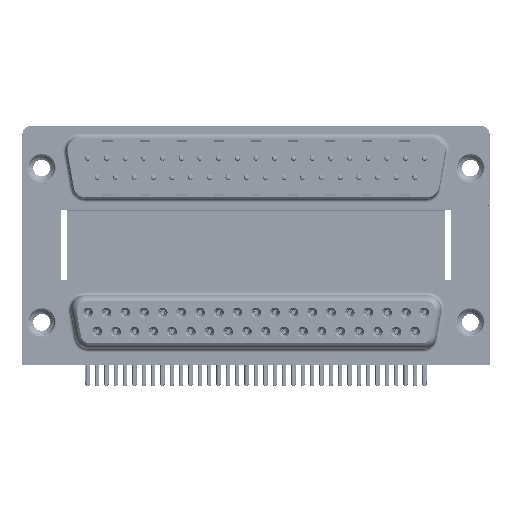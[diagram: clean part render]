
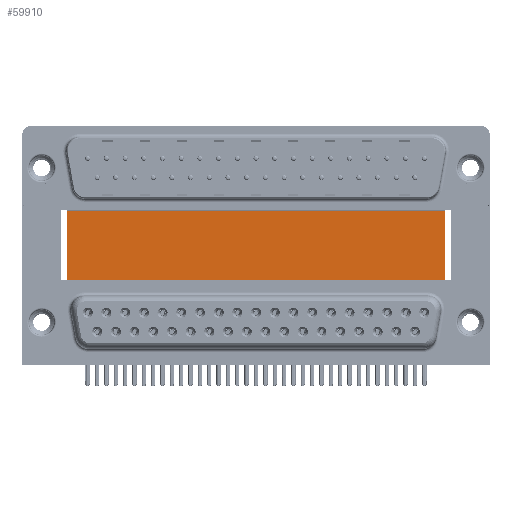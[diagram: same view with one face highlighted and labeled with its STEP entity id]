
A CAD part, top view. The second image highlights one B-rep face of the part: STEP entity #59910.
In plain terms, the highlighted planar face has unit normal (0, 0, 1).
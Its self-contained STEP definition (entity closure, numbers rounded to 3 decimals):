
#2184 = EDGE_CURVE ( 'NONE', #16338, #67508, #48367, .T. ) ;
#2792 = PLANE ( 'NONE',  #22619 ) ;
#4740 = VECTOR ( 'NONE', #37841, 1000. ) ;
#6722 = VECTOR ( 'NONE', #44417, 1000. ) ;
#8846 = DIRECTION ( 'NONE',  ( 0., 0., -1. ) ) ;
#11125 = ORIENTED_EDGE ( 'NONE', *, *, #2184, .F. ) ;
#14755 = EDGE_LOOP ( 'NONE', ( #58675, #37322, #11125, #35651 ) ) ;
#16338 = VERTEX_POINT ( 'NONE', #57147 ) ;
#21140 = LINE ( 'NONE', #42816, #4740 ) ;
#22619 = AXIS2_PLACEMENT_3D ( 'NONE', #57122, #8846, #56070 ) ;
#25188 = VERTEX_POINT ( 'NONE', #70006 ) ;
#33525 = CARTESIAN_POINT ( 'NONE',  ( 59.71, 16.585, -12. ) ) ;
#35651 = ORIENTED_EDGE ( 'NONE', *, *, #64796, .T. ) ;
#37322 = ORIENTED_EDGE ( 'NONE', *, *, #51460, .F. ) ;
#37841 = DIRECTION ( 'NONE',  ( 0., -1., 0. ) ) ;
#39160 = CARTESIAN_POINT ( 'NONE',  ( 59.71, 16.585, -12. ) ) ;
#41349 = CARTESIAN_POINT ( 'NONE',  ( 3.79, -3.735, -12. ) ) ;
#42816 = CARTESIAN_POINT ( 'NONE',  ( 3.79, 16.585, -12. ) ) ;
#43095 = CARTESIAN_POINT ( 'NONE',  ( 3.79, -3.735, -12. ) ) ;
#44417 = DIRECTION ( 'NONE',  ( 1., 0., 0. ) ) ;
#46168 = EDGE_CURVE ( 'NONE', #57973, #25188, #68975, .T. ) ;
#46302 = DIRECTION ( 'NONE',  ( 1., 0., 0. ) ) ;
#48367 = LINE ( 'NONE', #64647, #6722 ) ;
#51460 = EDGE_CURVE ( 'NONE', #67508, #25188, #64736, .T. ) ;
#54502 = VECTOR ( 'NONE', #65090, 1000. ) ;
#56070 = DIRECTION ( 'NONE',  ( -1., 0., 0. ) ) ;
#57122 = CARTESIAN_POINT ( 'NONE',  ( 3.79, 16.585, -12. ) ) ;
#57147 = CARTESIAN_POINT ( 'NONE',  ( 3.79, 16.585, -12. ) ) ;
#57596 = VECTOR ( 'NONE', #46302, 1000. ) ;
#57973 = VERTEX_POINT ( 'NONE', #43095 ) ;
#58675 = ORIENTED_EDGE ( 'NONE', *, *, #46168, .T. ) ;
#59910 = ADVANCED_FACE ( 'NONE', ( #68116 ), #2792, .F. ) ;
#64647 = CARTESIAN_POINT ( 'NONE',  ( 3.79, 16.585, -12. ) ) ;
#64736 = LINE ( 'NONE', #33525, #54502 ) ;
#64796 = EDGE_CURVE ( 'NONE', #16338, #57973, #21140, .T. ) ;
#65090 = DIRECTION ( 'NONE',  ( 0., -1., 0. ) ) ;
#67508 = VERTEX_POINT ( 'NONE', #39160 ) ;
#68116 = FACE_OUTER_BOUND ( 'NONE', #14755, .T. ) ;
#68975 = LINE ( 'NONE', #41349, #57596 ) ;
#70006 = CARTESIAN_POINT ( 'NONE',  ( 59.71, -3.735, -12. ) ) ;
